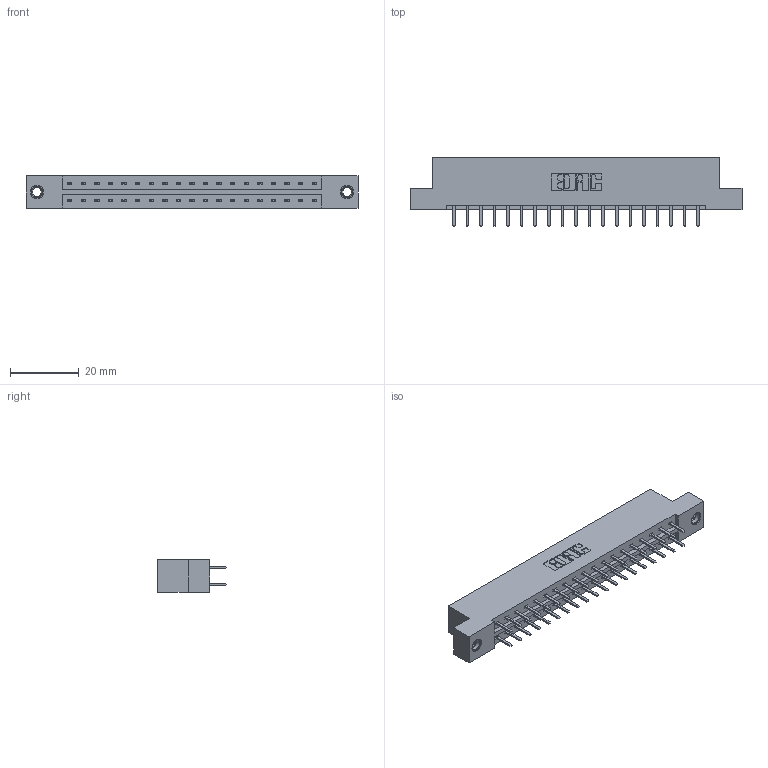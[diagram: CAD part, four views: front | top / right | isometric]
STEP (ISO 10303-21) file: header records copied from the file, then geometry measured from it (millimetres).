
FILE_DESCRIPTION (( 'STEP AP203' ), '1' );
FILE_NAME ('833-038-520-207.STEP', '2020-06-03T06:22:28', ( '' ), ( '' ), 'SwSTEP 2.0', 'SolidWorks 2020', '' );
FILE_SCHEMA (( 'CONFIG_CONTROL_DESIGN' ));
Length unit declared in the file: inch
Products named in the file (4): 345-292-001_345-293-120; 345-250-001_345-250-005-103; 833 Part_Flush - .156 Dia - TI; 833-038-520-207
Assembly tree (41 placements, depth 2):
  833-038-520-207
    833 Part_Flush - .156 Dia - TI
    345-292-001_345-293-120  x38
    345-250-001_345-250-005-103  x2
Bounding box: 96.82 x 20.02 x 9.4 mm (x, y, z)
Volume: 9639.9 mm3; surface area: 11139.6 mm2
Topology: 41 solids, 41 shells, 2302 faces, 6641 edges, 4318 vertices
Faces by surface type: plane 1546, cylinder 740, cone 12, torus 4
Entity records: 16498 total; most frequent: CARTESIAN_POINT 2757, ORIENTED_EDGE 2674, DIRECTION 2415, EDGE_CURVE 1337, VECTOR 1185, LINE 1185, VERTEX_POINT 884, AXIS2_PLACEMENT_3D 615
